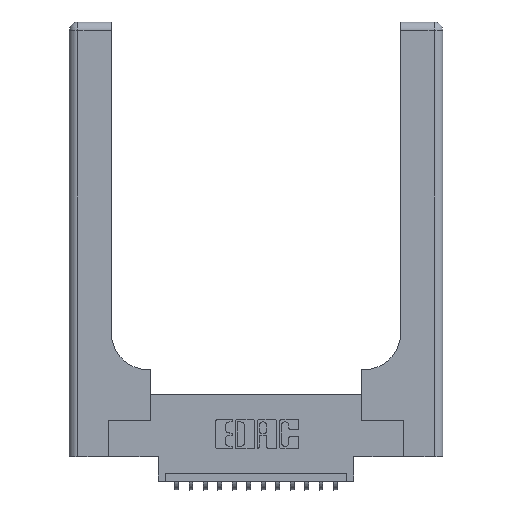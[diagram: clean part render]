
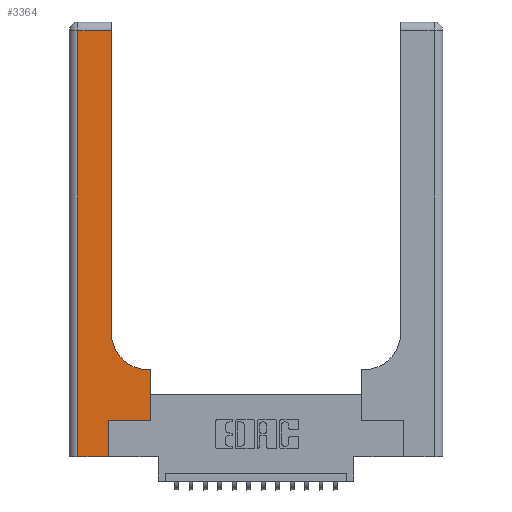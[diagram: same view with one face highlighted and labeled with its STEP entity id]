
A CAD part, top view. The second image highlights one B-rep face of the part: STEP entity #3364.
In plain terms, the highlighted planar face has unit normal (0, 0, 1).
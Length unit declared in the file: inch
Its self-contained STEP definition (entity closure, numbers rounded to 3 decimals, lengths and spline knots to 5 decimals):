
#38 = CARTESIAN_POINT ( 'NONE',  ( 0.06, 3., 0.37 ) ) ;
#517 = CARTESIAN_POINT ( 'NONE',  ( 0.269, 0., 0.37 ) ) ;
#612 = VECTOR ( 'NONE', #8926, 39.37008 ) ;
#1042 = LINE ( 'NONE', #6890, #16607 ) ;
#1052 = VERTEX_POINT ( 'NONE', #8026 ) ;
#1450 = EDGE_CURVE ( 'NONE', #11233, #9324, #8651, .T. ) ;
#1584 = DIRECTION ( 'NONE',  ( 1., 0., 0. ) ) ;
#1720 = PLANE ( 'NONE',  #16355 ) ;
#1894 = CARTESIAN_POINT ( 'NONE',  ( 0.06, 0., 0.37 ) ) ;
#1907 = EDGE_CURVE ( 'NONE', #14909, #15663, #1042, .T. ) ;
#2227 = EDGE_CURVE ( 'NONE', #12405, #15014, #12135, .T. ) ;
#2246 = VERTEX_POINT ( 'NONE', #2310 ) ;
#2310 = CARTESIAN_POINT ( 'NONE',  ( 0.2915, 0.85, 0.37 ) ) ;
#2575 = ORIENTED_EDGE ( 'NONE', *, *, #2227, .T. ) ;
#2676 = CARTESIAN_POINT ( 'NONE',  ( 0.269, 0.25, 0.37 ) ) ;
#2849 = VECTOR ( 'NONE', #11035, 39.37008 ) ;
#2871 = EDGE_CURVE ( 'NONE', #15014, #1052, #14368, .T. ) ;
#2954 = CARTESIAN_POINT ( 'NONE',  ( 0.06, 2.94, 0.37 ) ) ;
#3144 = DIRECTION ( 'NONE',  ( 0., 0., -1. ) ) ;
#3285 = VECTOR ( 'NONE', #10700, 39.37008 ) ;
#3364 = ADVANCED_FACE ( 'NONE', ( #14570 ), #1720, .F. ) ;
#3739 = EDGE_CURVE ( 'NONE', #9324, #12405, #12787, .T. ) ;
#5368 = EDGE_CURVE ( 'NONE', #15663, #15066, #5376, .T. ) ;
#5370 = DIRECTION ( 'NONE',  ( 1., 0., 0. ) ) ;
#5376 = LINE ( 'NONE', #38, #6286 ) ;
#5653 = CARTESIAN_POINT ( 'NONE',  ( 0.269, 0.25, 0.37 ) ) ;
#5885 = CARTESIAN_POINT ( 'NONE',  ( 0., 3., 0.37 ) ) ;
#6286 = VECTOR ( 'NONE', #10096, 39.37008 ) ;
#6890 = CARTESIAN_POINT ( 'NONE',  ( 0., 2.94, 0.37 ) ) ;
#7101 = VECTOR ( 'NONE', #17405, 39.37008 ) ;
#7901 = EDGE_LOOP ( 'NONE', ( #14660, #13728, #15494, #9996, #15794, #11946, #2575, #8589, #11959 ) ) ;
#8026 = CARTESIAN_POINT ( 'NONE',  ( 0.5415, 0.6, 0.37 ) ) ;
#8433 = CARTESIAN_POINT ( 'NONE',  ( 0.2915, 0.6, 0.37 ) ) ;
#8589 = ORIENTED_EDGE ( 'NONE', *, *, #2871, .T. ) ;
#8603 = EDGE_CURVE ( 'NONE', #15066, #11233, #14844, .T. ) ;
#8651 = LINE ( 'NONE', #11669, #612 ) ;
#8926 = DIRECTION ( 'NONE',  ( 0., 1., 0. ) ) ;
#9324 = VERTEX_POINT ( 'NONE', #5653 ) ;
#9996 = ORIENTED_EDGE ( 'NONE', *, *, #8603, .T. ) ;
#10096 = DIRECTION ( 'NONE',  ( 0., -1., 0. ) ) ;
#10183 = CARTESIAN_POINT ( 'NONE',  ( 0., 0., 0.37 ) ) ;
#10390 = AXIS2_PLACEMENT_3D ( 'NONE', #17299, #3144, #11691 ) ;
#10700 = DIRECTION ( 'NONE',  ( 0., 1., 0. ) ) ;
#11035 = DIRECTION ( 'NONE',  ( -1., 0., 0. ) ) ;
#11233 = VERTEX_POINT ( 'NONE', #517 ) ;
#11431 = EDGE_CURVE ( 'NONE', #1052, #2246, #11847, .T. ) ;
#11669 = CARTESIAN_POINT ( 'NONE',  ( 0.269, 0., 0.37 ) ) ;
#11691 = DIRECTION ( 'NONE',  ( 1., 0., 0. ) ) ;
#11800 = CARTESIAN_POINT ( 'NONE',  ( 0.2915, 3., 0.37 ) ) ;
#11847 = CIRCLE ( 'NONE', #10390, 0.25 ) ;
#11946 = ORIENTED_EDGE ( 'NONE', *, *, #3739, .T. ) ;
#11959 = ORIENTED_EDGE ( 'NONE', *, *, #11431, .T. ) ;
#12135 = LINE ( 'NONE', #13543, #3285 ) ;
#12405 = VERTEX_POINT ( 'NONE', #12654 ) ;
#12654 = CARTESIAN_POINT ( 'NONE',  ( 0.5585, 0.25, 0.37 ) ) ;
#12787 = LINE ( 'NONE', #2676, #15916 ) ;
#13067 = CARTESIAN_POINT ( 'NONE',  ( 0.5585, 0.6, 0.37 ) ) ;
#13529 = LINE ( 'NONE', #11800, #7101 ) ;
#13543 = CARTESIAN_POINT ( 'NONE',  ( 0.5585, 0.25, 0.37 ) ) ;
#13728 = ORIENTED_EDGE ( 'NONE', *, *, #1907, .T. ) ;
#13780 = EDGE_CURVE ( 'NONE', #2246, #14909, #13529, .T. ) ;
#14368 = LINE ( 'NONE', #8433, #2849 ) ;
#14570 = FACE_OUTER_BOUND ( 'NONE', #7901, .T. ) ;
#14660 = ORIENTED_EDGE ( 'NONE', *, *, #13780, .T. ) ;
#14819 = VECTOR ( 'NONE', #1584, 39.37008 ) ;
#14844 = LINE ( 'NONE', #10183, #14819 ) ;
#14909 = VERTEX_POINT ( 'NONE', #15817 ) ;
#15014 = VERTEX_POINT ( 'NONE', #13067 ) ;
#15066 = VERTEX_POINT ( 'NONE', #1894 ) ;
#15494 = ORIENTED_EDGE ( 'NONE', *, *, #5368, .T. ) ;
#15653 = DIRECTION ( 'NONE',  ( -1., 0., 0. ) ) ;
#15663 = VERTEX_POINT ( 'NONE', #2954 ) ;
#15794 = ORIENTED_EDGE ( 'NONE', *, *, #1450, .T. ) ;
#15817 = CARTESIAN_POINT ( 'NONE',  ( 0.2915, 2.94, 0.37 ) ) ;
#15916 = VECTOR ( 'NONE', #5370, 39.37008 ) ;
#16355 = AXIS2_PLACEMENT_3D ( 'NONE', #5885, #17259, #17318 ) ;
#16607 = VECTOR ( 'NONE', #15653, 39.37008 ) ;
#17259 = DIRECTION ( 'NONE',  ( 0., 0., -1. ) ) ;
#17299 = CARTESIAN_POINT ( 'NONE',  ( 0.5415, 0.85, 0.37 ) ) ;
#17318 = DIRECTION ( 'NONE',  ( -1., 0., 0. ) ) ;
#17405 = DIRECTION ( 'NONE',  ( 0., 1., 0. ) ) ;
